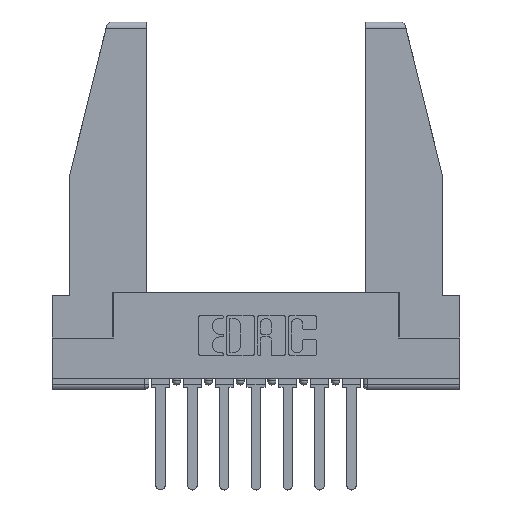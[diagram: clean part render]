
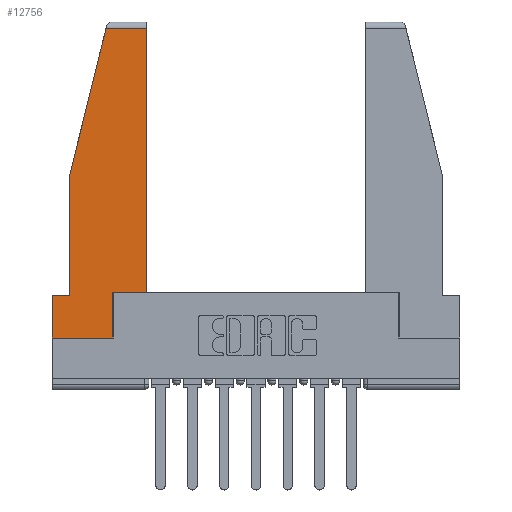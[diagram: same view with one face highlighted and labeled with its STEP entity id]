
A CAD part, top view. The second image highlights one B-rep face of the part: STEP entity #12756.
In plain terms, the highlighted planar face has unit normal (0, 0, 1).
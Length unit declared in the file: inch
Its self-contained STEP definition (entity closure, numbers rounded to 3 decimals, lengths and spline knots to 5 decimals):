
#77 = VERTEX_POINT ( 'NONE', #12354 ) ;
#85 = CARTESIAN_POINT ( 'NONE',  ( 0., 0.21, 0. ) ) ;
#661 = PLANE ( 'NONE',  #11712 ) ;
#715 = CARTESIAN_POINT ( 'NONE',  ( 0.461, 1.52, 0. ) ) ;
#883 = VECTOR ( 'NONE', #10577, 39.37008 ) ;
#1251 = CARTESIAN_POINT ( 'NONE',  ( 0.461, 0.223, 0. ) ) ;
#1339 = VECTOR ( 'NONE', #12260, 39.37008 ) ;
#1390 = LINE ( 'NONE', #1251, #11135 ) ;
#1754 = EDGE_CURVE ( 'NONE', #5095, #8421, #10572, .T. ) ;
#2203 = DIRECTION ( 'NONE',  ( -0.239, -0.971, 0. ) ) ;
#2583 = EDGE_LOOP ( 'NONE', ( #8067, #7464, #10835, #7727, #5592, #10037, #8147, #3764, #9082 ) ) ;
#2726 = CARTESIAN_POINT ( 'NONE',  ( 0., 0., 0. ) ) ;
#2833 = EDGE_CURVE ( 'NONE', #4107, #77, #11687, .T. ) ;
#3096 = CARTESIAN_POINT ( 'NONE',  ( 0., 1.52, 0. ) ) ;
#3122 = VECTOR ( 'NONE', #10646, 39.37008 ) ;
#3244 = EDGE_CURVE ( 'NONE', #3915, #5095, #1390, .T. ) ;
#3605 = DIRECTION ( 'NONE',  ( 0., 1., 0. ) ) ;
#3764 = ORIENTED_EDGE ( 'NONE', *, *, #2833, .T. ) ;
#3829 = CARTESIAN_POINT ( 'NONE',  ( 0., 0.21, 0. ) ) ;
#3915 = VERTEX_POINT ( 'NONE', #9465 ) ;
#4060 = DIRECTION ( 'NONE',  ( 1., 0., 0. ) ) ;
#4098 = VERTEX_POINT ( 'NONE', #9993 ) ;
#4107 = VERTEX_POINT ( 'NONE', #10123 ) ;
#4410 = DIRECTION ( 'NONE',  ( 0., 1., 0. ) ) ;
#4745 = LINE ( 'NONE', #2726, #7932 ) ;
#4868 = EDGE_CURVE ( 'NONE', #11731, #11732, #12828, .T. ) ;
#4986 = CARTESIAN_POINT ( 'NONE',  ( 0.297, 0.223, 0. ) ) ;
#5095 = VERTEX_POINT ( 'NONE', #715 ) ;
#5146 = EDGE_CURVE ( 'NONE', #11593, #11731, #13491, .T. ) ;
#5592 = ORIENTED_EDGE ( 'NONE', *, *, #4868, .T. ) ;
#5844 = DIRECTION ( 'NONE',  ( 0., 0., 1. ) ) ;
#5988 = FACE_OUTER_BOUND ( 'NONE', #2583, .T. ) ;
#6069 = DIRECTION ( 'NONE',  ( 0., -1., 0. ) ) ;
#6684 = VECTOR ( 'NONE', #2203, 39.37008 ) ;
#6948 = LINE ( 'NONE', #4986, #9538 ) ;
#7024 = EDGE_CURVE ( 'NONE', #77, #3915, #6948, .T. ) ;
#7288 = CARTESIAN_POINT ( 'NONE',  ( 0.086, 0.8, 0. ) ) ;
#7464 = ORIENTED_EDGE ( 'NONE', *, *, #1754, .T. ) ;
#7727 = ORIENTED_EDGE ( 'NONE', *, *, #5146, .T. ) ;
#7932 = VECTOR ( 'NONE', #8194, 39.37008 ) ;
#8067 = ORIENTED_EDGE ( 'NONE', *, *, #3244, .T. ) ;
#8147 = ORIENTED_EDGE ( 'NONE', *, *, #9752, .T. ) ;
#8194 = DIRECTION ( 'NONE',  ( 1., 0., 0. ) ) ;
#8255 = CARTESIAN_POINT ( 'NONE',  ( 0.2636, 1.52, 0. ) ) ;
#8421 = VERTEX_POINT ( 'NONE', #8255 ) ;
#9082 = ORIENTED_EDGE ( 'NONE', *, *, #7024, .T. ) ;
#9327 = EDGE_CURVE ( 'NONE', #11732, #4098, #12373, .T. ) ;
#9465 = CARTESIAN_POINT ( 'NONE',  ( 0.461, 0.223, 0. ) ) ;
#9538 = VECTOR ( 'NONE', #11117, 39.37008 ) ;
#9752 = EDGE_CURVE ( 'NONE', #4098, #4107, #4745, .T. ) ;
#9993 = CARTESIAN_POINT ( 'NONE',  ( 0., 0., 0. ) ) ;
#10037 = ORIENTED_EDGE ( 'NONE', *, *, #9327, .T. ) ;
#10123 = CARTESIAN_POINT ( 'NONE',  ( 0.297, 0., 0. ) ) ;
#10168 = CARTESIAN_POINT ( 'NONE',  ( 0., 0., 0. ) ) ;
#10214 = CARTESIAN_POINT ( 'NONE',  ( 0.086, 0.8, 0. ) ) ;
#10563 = LINE ( 'NONE', #10637, #6684 ) ;
#10572 = LINE ( 'NONE', #3096, #3122 ) ;
#10577 = DIRECTION ( 'NONE',  ( -1., 0., 0. ) ) ;
#10637 = CARTESIAN_POINT ( 'NONE',  ( 0.271, 1.55, 0. ) ) ;
#10646 = DIRECTION ( 'NONE',  ( -1., 0., 0. ) ) ;
#10679 = CARTESIAN_POINT ( 'NONE',  ( 0.297, 0., 0. ) ) ;
#10835 = ORIENTED_EDGE ( 'NONE', *, *, #13391, .T. ) ;
#11117 = DIRECTION ( 'NONE',  ( 1., 0., 0. ) ) ;
#11135 = VECTOR ( 'NONE', #4410, 39.37008 ) ;
#11593 = VERTEX_POINT ( 'NONE', #7288 ) ;
#11659 = CARTESIAN_POINT ( 'NONE',  ( 0., 0.21, 0. ) ) ;
#11687 = LINE ( 'NONE', #10679, #13497 ) ;
#11712 = AXIS2_PLACEMENT_3D ( 'NONE', #10168, #5844, #4060 ) ;
#11731 = VERTEX_POINT ( 'NONE', #11856 ) ;
#11732 = VERTEX_POINT ( 'NONE', #3829 ) ;
#11856 = CARTESIAN_POINT ( 'NONE',  ( 0.086, 0.21, 0. ) ) ;
#12260 = DIRECTION ( 'NONE',  ( 0., -1., 0. ) ) ;
#12354 = CARTESIAN_POINT ( 'NONE',  ( 0.297, 0.223, 0. ) ) ;
#12373 = LINE ( 'NONE', #85, #12494 ) ;
#12494 = VECTOR ( 'NONE', #6069, 39.37008 ) ;
#12756 = ADVANCED_FACE ( 'NONE', ( #5988 ), #661, .T. ) ;
#12828 = LINE ( 'NONE', #11659, #883 ) ;
#13391 = EDGE_CURVE ( 'NONE', #8421, #11593, #10563, .T. ) ;
#13491 = LINE ( 'NONE', #10214, #1339 ) ;
#13497 = VECTOR ( 'NONE', #3605, 39.37008 ) ;
